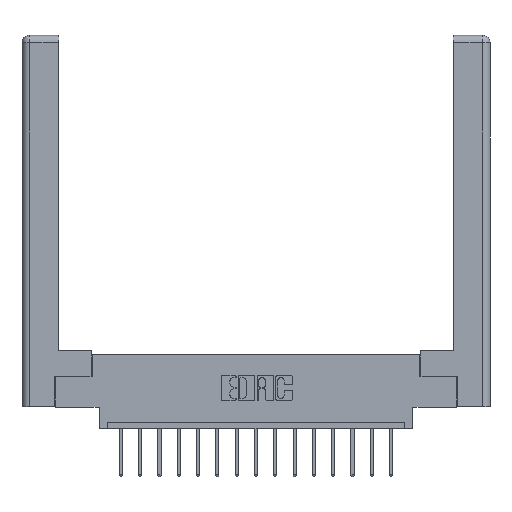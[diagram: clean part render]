
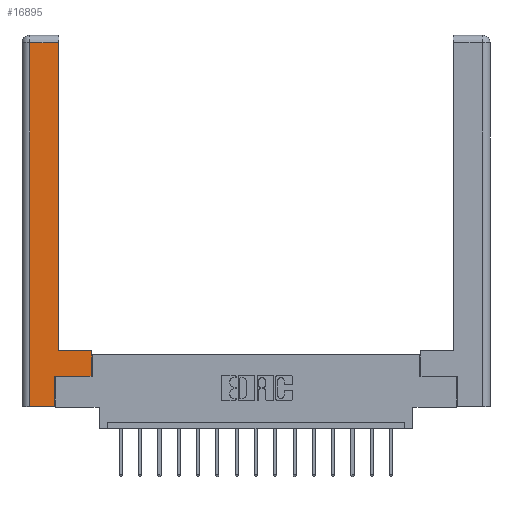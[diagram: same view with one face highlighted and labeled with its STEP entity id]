
A CAD part, top view. The second image highlights one B-rep face of the part: STEP entity #16895.
In plain terms, the highlighted planar face has unit normal (0, 0, 1).
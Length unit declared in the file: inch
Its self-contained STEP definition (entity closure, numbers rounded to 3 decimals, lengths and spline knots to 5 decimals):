
#542 = FACE_OUTER_BOUND ( 'NONE', #3405, .T. ) ;
#562 = CARTESIAN_POINT ( 'NONE',  ( 0.265, 0., 0. ) ) ;
#625 = VECTOR ( 'NONE', #16957, 39.37008 ) ;
#636 = VECTOR ( 'NONE', #12598, 39.37008 ) ;
#902 = CARTESIAN_POINT ( 'NONE',  ( 0.565, 0.245, 0. ) ) ;
#929 = VERTEX_POINT ( 'NONE', #12686 ) ;
#1124 = CARTESIAN_POINT ( 'NONE',  ( 0.265, 0., 0. ) ) ;
#1295 = LINE ( 'NONE', #1124, #12489 ) ;
#1437 = CARTESIAN_POINT ( 'NONE',  ( 0.295, 3., 0. ) ) ;
#1843 = EDGE_CURVE ( 'NONE', #3328, #1953, #17053, .T. ) ;
#1953 = VERTEX_POINT ( 'NONE', #17247 ) ;
#2076 = EDGE_CURVE ( 'NONE', #7195, #3328, #2883, .T. ) ;
#2151 = EDGE_CURVE ( 'NONE', #1953, #6847, #14461, .T. ) ;
#2883 = LINE ( 'NONE', #15964, #3926 ) ;
#3123 = ORIENTED_EDGE ( 'NONE', *, *, #2076, .T. ) ;
#3328 = VERTEX_POINT ( 'NONE', #9355 ) ;
#3405 = EDGE_LOOP ( 'NONE', ( #11439, #4761, #7883, #12348, #7920, #5957, #3123, #13330 ) ) ;
#3926 = VECTOR ( 'NONE', #10571, 39.37008 ) ;
#4729 = LINE ( 'NONE', #902, #5984 ) ;
#4761 = ORIENTED_EDGE ( 'NONE', *, *, #12251, .T. ) ;
#5957 = ORIENTED_EDGE ( 'NONE', *, *, #8450, .T. ) ;
#5984 = VECTOR ( 'NONE', #11663, 39.37008 ) ;
#6067 = LINE ( 'NONE', #14313, #7930 ) ;
#6468 = CARTESIAN_POINT ( 'NONE',  ( 0.0615, 2.94, 0. ) ) ;
#6847 = VERTEX_POINT ( 'NONE', #8766 ) ;
#7195 = VERTEX_POINT ( 'NONE', #17417 ) ;
#7237 = CARTESIAN_POINT ( 'NONE',  ( 0.265, 0.245, 0. ) ) ;
#7357 = LINE ( 'NONE', #16614, #636 ) ;
#7564 = DIRECTION ( 'NONE',  ( 0., 0., -1. ) ) ;
#7883 = ORIENTED_EDGE ( 'NONE', *, *, #14603, .T. ) ;
#7920 = ORIENTED_EDGE ( 'NONE', *, *, #14101, .T. ) ;
#7930 = VECTOR ( 'NONE', #11567, 39.37008 ) ;
#7941 = VERTEX_POINT ( 'NONE', #15346 ) ;
#8365 = AXIS2_PLACEMENT_3D ( 'NONE', #11652, #7564, #17009 ) ;
#8450 = EDGE_CURVE ( 'NONE', #929, #7195, #4729, .T. ) ;
#8766 = CARTESIAN_POINT ( 'NONE',  ( 0.295, 2.94, 0. ) ) ;
#8924 = VERTEX_POINT ( 'NONE', #6468 ) ;
#9118 = VERTEX_POINT ( 'NONE', #562 ) ;
#9355 = CARTESIAN_POINT ( 'NONE',  ( 0.565, 0.45, 0. ) ) ;
#9569 = DIRECTION ( 'NONE',  ( 0., 1., 0. ) ) ;
#9584 = EDGE_CURVE ( 'NONE', #7941, #9118, #1295, .T. ) ;
#9593 = VECTOR ( 'NONE', #16490, 39.37008 ) ;
#10540 = DIRECTION ( 'NONE',  ( 1., 0., 0. ) ) ;
#10571 = DIRECTION ( 'NONE',  ( 0., 1., 0. ) ) ;
#11062 = LINE ( 'NONE', #7237, #9593 ) ;
#11439 = ORIENTED_EDGE ( 'NONE', *, *, #2151, .T. ) ;
#11567 = DIRECTION ( 'NONE',  ( -1., 0., 0. ) ) ;
#11652 = CARTESIAN_POINT ( 'NONE',  ( 0., 0., 0. ) ) ;
#11663 = DIRECTION ( 'NONE',  ( 1., 0., 0. ) ) ;
#12251 = EDGE_CURVE ( 'NONE', #6847, #8924, #6067, .T. ) ;
#12348 = ORIENTED_EDGE ( 'NONE', *, *, #9584, .T. ) ;
#12489 = VECTOR ( 'NONE', #10540, 39.37008 ) ;
#12598 = DIRECTION ( 'NONE',  ( 0., -1., 0. ) ) ;
#12686 = CARTESIAN_POINT ( 'NONE',  ( 0.265, 0.245, 0. ) ) ;
#13330 = ORIENTED_EDGE ( 'NONE', *, *, #1843, .T. ) ;
#14101 = EDGE_CURVE ( 'NONE', #9118, #929, #11062, .T. ) ;
#14270 = PLANE ( 'NONE',  #8365 ) ;
#14313 = CARTESIAN_POINT ( 'NONE',  ( 0.0615, 2.94, 0. ) ) ;
#14461 = LINE ( 'NONE', #1437, #16396 ) ;
#14603 = EDGE_CURVE ( 'NONE', #8924, #7941, #7357, .T. ) ;
#15346 = CARTESIAN_POINT ( 'NONE',  ( 0.0615, 0., 0. ) ) ;
#15526 = CARTESIAN_POINT ( 'NONE',  ( 0.295, 0.45, 0. ) ) ;
#15964 = CARTESIAN_POINT ( 'NONE',  ( 0.565, 0.45, 0. ) ) ;
#16396 = VECTOR ( 'NONE', #9569, 39.37008 ) ;
#16490 = DIRECTION ( 'NONE',  ( 0., 1., 0. ) ) ;
#16614 = CARTESIAN_POINT ( 'NONE',  ( 0.0615, 0., 0. ) ) ;
#16895 = ADVANCED_FACE ( 'NONE', ( #542 ), #14270, .F. ) ;
#16957 = DIRECTION ( 'NONE',  ( -1., 0., 0. ) ) ;
#17009 = DIRECTION ( 'NONE',  ( -1., 0., 0. ) ) ;
#17053 = LINE ( 'NONE', #15526, #625 ) ;
#17247 = CARTESIAN_POINT ( 'NONE',  ( 0.295, 0.45, 0. ) ) ;
#17417 = CARTESIAN_POINT ( 'NONE',  ( 0.565, 0.245, 0. ) ) ;
